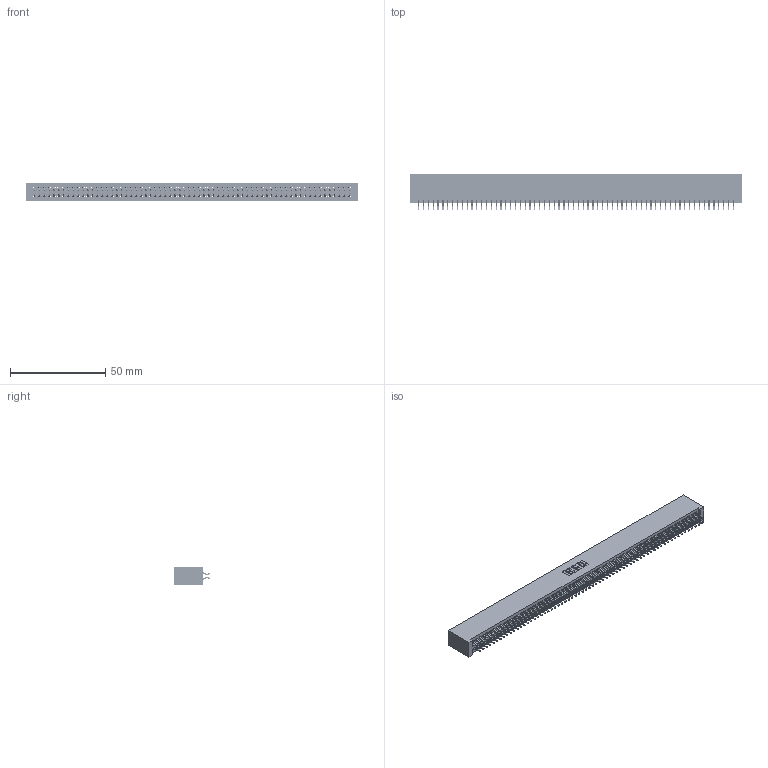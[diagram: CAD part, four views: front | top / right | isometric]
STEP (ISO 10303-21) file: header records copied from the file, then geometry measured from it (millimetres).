
FILE_DESCRIPTION (( 'STEP AP203' ), '1' );
FILE_NAME ('395-132-556-201.STEP', '2018-12-04T23:38:36', ( '' ), ( '' ), 'SwSTEP 2.0', 'SolidWorks 2016', '' );
FILE_SCHEMA (( 'CONFIG_CONTROL_DESIGN' ));
Length unit declared in the file: inch
Products named in the file (3): 395-132-556-201; 345 Part_No Mounting Lugs; 345-292-001_556 Tail
Assembly tree (133 placements, depth 2):
  395-132-556-201
    345 Part_No Mounting Lugs
    345-292-001_556 Tail  x132
Bounding box: 174.24 x 19.24 x 9.4 mm (x, y, z)
Volume: 17759.7 mm3; surface area: 26904.4 mm2
Topology: 133 solids, 133 shells, 7510 faces, 22361 edges, 14730 vertices
Faces by surface type: plane 4960, cylinder 2550
Entity records: 48497 total; most frequent: CARTESIAN_POINT 8120, ORIENTED_EDGE 8042, DIRECTION 7113, EDGE_CURVE 4021, LINE 3625, VECTOR 3625, VERTEX_POINT 2678, AXIS2_PLACEMENT_3D 1744
